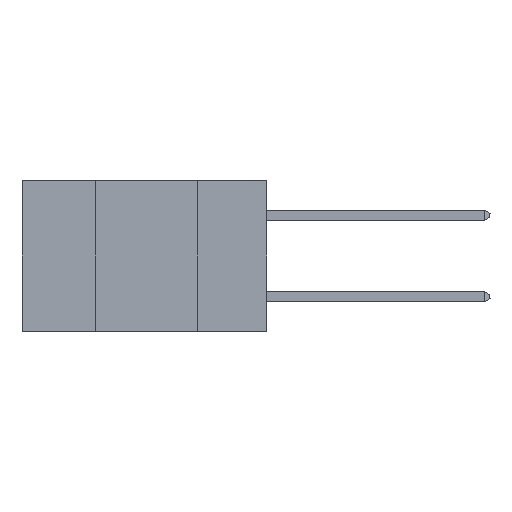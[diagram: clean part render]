
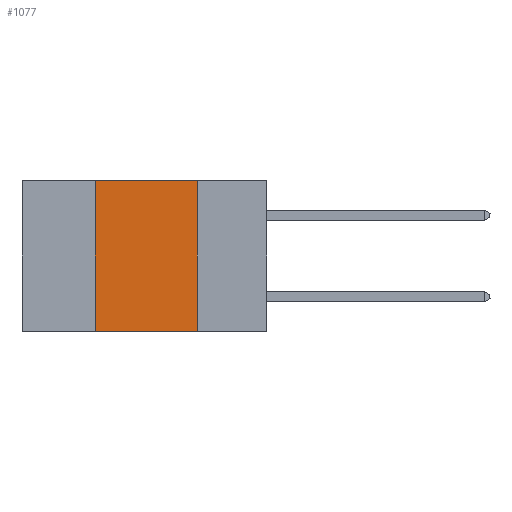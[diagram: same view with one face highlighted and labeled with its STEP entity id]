
A CAD part, left-side view. The second image highlights one B-rep face of the part: STEP entity #1077.
In plain terms, the highlighted planar face has unit normal (-1, 0, 0).
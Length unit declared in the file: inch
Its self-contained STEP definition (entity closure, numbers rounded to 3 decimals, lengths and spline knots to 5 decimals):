
#1077 = ADVANCED_FACE ( 'NONE', ( #36578 ), #36874, .F. ) ;
#2139 = CARTESIAN_POINT ( 'NONE',  ( 0., 0.6, 0. ) ) ;
#2699 = EDGE_CURVE ( 'NONE', #18358, #39433, #13332, .T. ) ;
#3644 = CARTESIAN_POINT ( 'NONE',  ( 0., 0.6, -0.37 ) ) ;
#4497 = CARTESIAN_POINT ( 'NONE',  ( 0., 0.17, 0. ) ) ;
#5269 = LINE ( 'NONE', #3644, #12725 ) ;
#7795 = AXIS2_PLACEMENT_3D ( 'NONE', #2139, #18123, #40028 ) ;
#8864 = LINE ( 'NONE', #22274, #24638 ) ;
#9787 = VERTEX_POINT ( 'NONE', #18542 ) ;
#10832 = CARTESIAN_POINT ( 'NONE',  ( 0., 0.17, -0.37 ) ) ;
#12725 = VECTOR ( 'NONE', #13090, 39.37008 ) ;
#13090 = DIRECTION ( 'NONE',  ( 0., -1., 0. ) ) ;
#13332 = LINE ( 'NONE', #35692, #29073 ) ;
#14641 = ORIENTED_EDGE ( 'NONE', *, *, #2699, .F. ) ;
#15635 = ORIENTED_EDGE ( 'NONE', *, *, #35234, .F. ) ;
#16202 = VERTEX_POINT ( 'NONE', #25335 ) ;
#18123 = DIRECTION ( 'NONE',  ( 1., 0., 0. ) ) ;
#18358 = VERTEX_POINT ( 'NONE', #4497 ) ;
#18542 = CARTESIAN_POINT ( 'NONE',  ( 0., 0.42, -0.37 ) ) ;
#22274 = CARTESIAN_POINT ( 'NONE',  ( 0., 0.42, 0. ) ) ;
#23016 = ORIENTED_EDGE ( 'NONE', *, *, #33946, .F. ) ;
#23583 = EDGE_LOOP ( 'NONE', ( #14641, #23016, #15635, #25963 ) ) ;
#24638 = VECTOR ( 'NONE', #25434, 39.37008 ) ;
#25335 = CARTESIAN_POINT ( 'NONE',  ( 0., 0.42, 0. ) ) ;
#25377 = DIRECTION ( 'NONE',  ( 0., -1., 0. ) ) ;
#25434 = DIRECTION ( 'NONE',  ( 0., 0., 1. ) ) ;
#25963 = ORIENTED_EDGE ( 'NONE', *, *, #26813, .T. ) ;
#26813 = EDGE_CURVE ( 'NONE', #9787, #39433, #5269, .T. ) ;
#29073 = VECTOR ( 'NONE', #38850, 39.37008 ) ;
#29600 = VECTOR ( 'NONE', #25377, 39.37008 ) ;
#30569 = LINE ( 'NONE', #37870, #29600 ) ;
#33946 = EDGE_CURVE ( 'NONE', #16202, #18358, #30569, .T. ) ;
#35234 = EDGE_CURVE ( 'NONE', #9787, #16202, #8864, .T. ) ;
#35692 = CARTESIAN_POINT ( 'NONE',  ( 0., 0.17, 0. ) ) ;
#36578 = FACE_OUTER_BOUND ( 'NONE', #23583, .T. ) ;
#36874 = PLANE ( 'NONE',  #7795 ) ;
#37870 = CARTESIAN_POINT ( 'NONE',  ( 0., 0.6, 0. ) ) ;
#38850 = DIRECTION ( 'NONE',  ( 0., 0., -1. ) ) ;
#39433 = VERTEX_POINT ( 'NONE', #10832 ) ;
#40028 = DIRECTION ( 'NONE',  ( 0., 0., -1. ) ) ;
